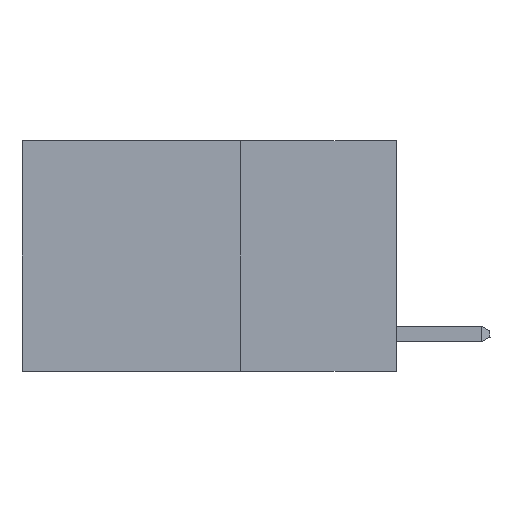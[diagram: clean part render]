
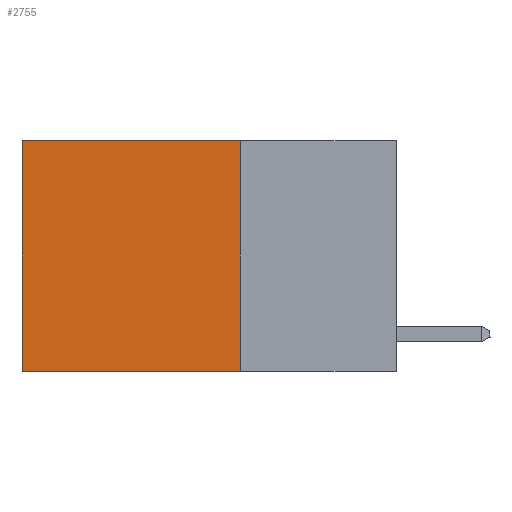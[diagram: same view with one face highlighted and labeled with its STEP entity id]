
A CAD part, left-side view. The second image highlights one B-rep face of the part: STEP entity #2755.
In plain terms, the highlighted planar face has unit normal (-1, 0, 0).
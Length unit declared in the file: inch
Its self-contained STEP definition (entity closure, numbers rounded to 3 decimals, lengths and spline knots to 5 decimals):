
#143 = VECTOR ( 'NONE', #354, 39.37008 ) ;
#354 = DIRECTION ( 'NONE',  ( 0., 1., 0. ) ) ;
#525 = CARTESIAN_POINT ( 'NONE',  ( 0.2625, 0.25, 0. ) ) ;
#878 = AXIS2_PLACEMENT_3D ( 'NONE', #8023, #3286, #4674 ) ;
#1177 = EDGE_CURVE ( 'NONE', #3036, #1810, #5684, .T. ) ;
#1207 = ORIENTED_EDGE ( 'NONE', *, *, #6159, .F. ) ;
#1693 = CARTESIAN_POINT ( 'NONE',  ( 0.2625, 0.6, 0. ) ) ;
#1810 = VERTEX_POINT ( 'NONE', #4766 ) ;
#1868 = LINE ( 'NONE', #6663, #1987 ) ;
#1987 = VECTOR ( 'NONE', #3893, 39.37008 ) ;
#2567 = EDGE_CURVE ( 'NONE', #8434, #1810, #4442, .T. ) ;
#2755 = ADVANCED_FACE ( 'NONE', ( #4757 ), #5403, .F. ) ;
#3036 = VERTEX_POINT ( 'NONE', #6525 ) ;
#3286 = DIRECTION ( 'NONE',  ( 1., 0., 0. ) ) ;
#3860 = EDGE_LOOP ( 'NONE', ( #8137, #7885, #1207, #6445 ) ) ;
#3893 = DIRECTION ( 'NONE',  ( 0., 0., -1. ) ) ;
#4442 = LINE ( 'NONE', #1693, #6691 ) ;
#4563 = CARTESIAN_POINT ( 'NONE',  ( 0.2625, 0.6, 0. ) ) ;
#4674 = DIRECTION ( 'NONE',  ( 0., 0., -1. ) ) ;
#4757 = FACE_OUTER_BOUND ( 'NONE', #3860, .T. ) ;
#4766 = CARTESIAN_POINT ( 'NONE',  ( 0.2625, 0.6, -0.37 ) ) ;
#5031 = CARTESIAN_POINT ( 'NONE',  ( 0.2625, 0.25, -0.37 ) ) ;
#5043 = VECTOR ( 'NONE', #8493, 39.37008 ) ;
#5045 = DIRECTION ( 'NONE',  ( 0., 0., -1. ) ) ;
#5403 = PLANE ( 'NONE',  #878 ) ;
#5684 = LINE ( 'NONE', #5031, #143 ) ;
#6158 = EDGE_CURVE ( 'NONE', #8208, #8434, #6620, .T. ) ;
#6159 = EDGE_CURVE ( 'NONE', #8208, #3036, #1868, .T. ) ;
#6445 = ORIENTED_EDGE ( 'NONE', *, *, #6158, .T. ) ;
#6525 = CARTESIAN_POINT ( 'NONE',  ( 0.2625, 0.25, -0.37 ) ) ;
#6620 = LINE ( 'NONE', #7810, #5043 ) ;
#6663 = CARTESIAN_POINT ( 'NONE',  ( 0.2625, 0.25, 0. ) ) ;
#6691 = VECTOR ( 'NONE', #5045, 39.37008 ) ;
#7810 = CARTESIAN_POINT ( 'NONE',  ( 0.2625, 0.25, 0. ) ) ;
#7885 = ORIENTED_EDGE ( 'NONE', *, *, #1177, .F. ) ;
#8023 = CARTESIAN_POINT ( 'NONE',  ( 0.2625, 0.25, 0. ) ) ;
#8137 = ORIENTED_EDGE ( 'NONE', *, *, #2567, .T. ) ;
#8208 = VERTEX_POINT ( 'NONE', #525 ) ;
#8434 = VERTEX_POINT ( 'NONE', #4563 ) ;
#8493 = DIRECTION ( 'NONE',  ( 0., 1., 0. ) ) ;
